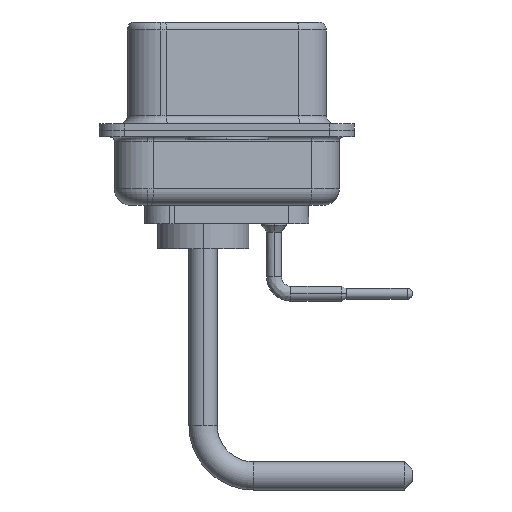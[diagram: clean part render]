
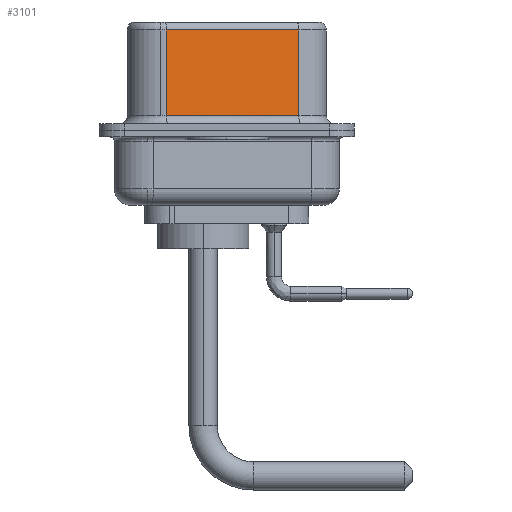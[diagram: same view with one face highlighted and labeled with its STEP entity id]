
A CAD part, left-side view. The second image highlights one B-rep face of the part: STEP entity #3101.
In plain terms, the highlighted planar face has unit normal (-0.985, -0.174, 0).
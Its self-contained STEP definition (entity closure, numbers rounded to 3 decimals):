
#41 = LINE ( 'NONE', #14081, #8927 ) ;
#367 = VERTEX_POINT ( 'NONE', #11561 ) ;
#3101 = ADVANCED_FACE ( 'NONE', ( #5564 ), #17822, .F. ) ;
#4413 = CARTESIAN_POINT ( 'NONE',  ( 3.73, 3.628, 0.9 ) ) ;
#4514 = LINE ( 'NONE', #13216, #15485 ) ;
#4767 = EDGE_CURVE ( 'NONE', #10844, #367, #41, .T. ) ;
#4911 = EDGE_CURVE ( 'NONE', #7190, #10844, #18078, .T. ) ;
#5314 = ORIENTED_EDGE ( 'NONE', *, *, #4767, .T. ) ;
#5564 = FACE_OUTER_BOUND ( 'NONE', #11743, .T. ) ;
#6135 = AXIS2_PLACEMENT_3D ( 'NONE', #19403, #19179, #16140 ) ;
#6625 = VERTEX_POINT ( 'NONE', #13470 ) ;
#7190 = VERTEX_POINT ( 'NONE', #20825 ) ;
#7607 = DIRECTION ( 'NONE',  ( 0.174, -0.985, 0. ) ) ;
#7826 = DIRECTION ( 'NONE',  ( 0., 0., -1. ) ) ;
#8927 = VECTOR ( 'NONE', #7607, 1000. ) ;
#10422 = LINE ( 'NONE', #15311, #19930 ) ;
#10844 = VERTEX_POINT ( 'NONE', #4413 ) ;
#11561 = CARTESIAN_POINT ( 'NONE',  ( 5.132, -4.322, 0.9 ) ) ;
#11743 = EDGE_LOOP ( 'NONE', ( #14066, #13584, #14761, #5314 ) ) ;
#12836 = VECTOR ( 'NONE', #7826, 1000. ) ;
#12848 = CARTESIAN_POINT ( 'NONE',  ( 3.73, 3.628, 6.52 ) ) ;
#13216 = CARTESIAN_POINT ( 'NONE',  ( 5.132, -4.322, 6.52 ) ) ;
#13470 = CARTESIAN_POINT ( 'NONE',  ( 5.132, -4.322, 6.02 ) ) ;
#13584 = ORIENTED_EDGE ( 'NONE', *, *, #20426, .T. ) ;
#14066 = ORIENTED_EDGE ( 'NONE', *, *, #15382, .F. ) ;
#14081 = CARTESIAN_POINT ( 'NONE',  ( 5.132, -4.322, 0.9 ) ) ;
#14761 = ORIENTED_EDGE ( 'NONE', *, *, #4911, .T. ) ;
#15311 = CARTESIAN_POINT ( 'NONE',  ( 5.132, -4.322, 6.02 ) ) ;
#15382 = EDGE_CURVE ( 'NONE', #6625, #367, #4514, .T. ) ;
#15485 = VECTOR ( 'NONE', #19706, 1000. ) ;
#15535 = DIRECTION ( 'NONE',  ( -0.174, 0.985, 0. ) ) ;
#16140 = DIRECTION ( 'NONE',  ( -0.174, 0.985, 0. ) ) ;
#17822 = PLANE ( 'NONE',  #6135 ) ;
#18078 = LINE ( 'NONE', #12848, #12836 ) ;
#19179 = DIRECTION ( 'NONE',  ( 0.985, 0.174, 0. ) ) ;
#19403 = CARTESIAN_POINT ( 'NONE',  ( 5.132, -4.322, 6.52 ) ) ;
#19706 = DIRECTION ( 'NONE',  ( 0., 0., -1. ) ) ;
#19930 = VECTOR ( 'NONE', #15535, 1000. ) ;
#20426 = EDGE_CURVE ( 'NONE', #6625, #7190, #10422, .T. ) ;
#20825 = CARTESIAN_POINT ( 'NONE',  ( 3.73, 3.628, 6.02 ) ) ;
